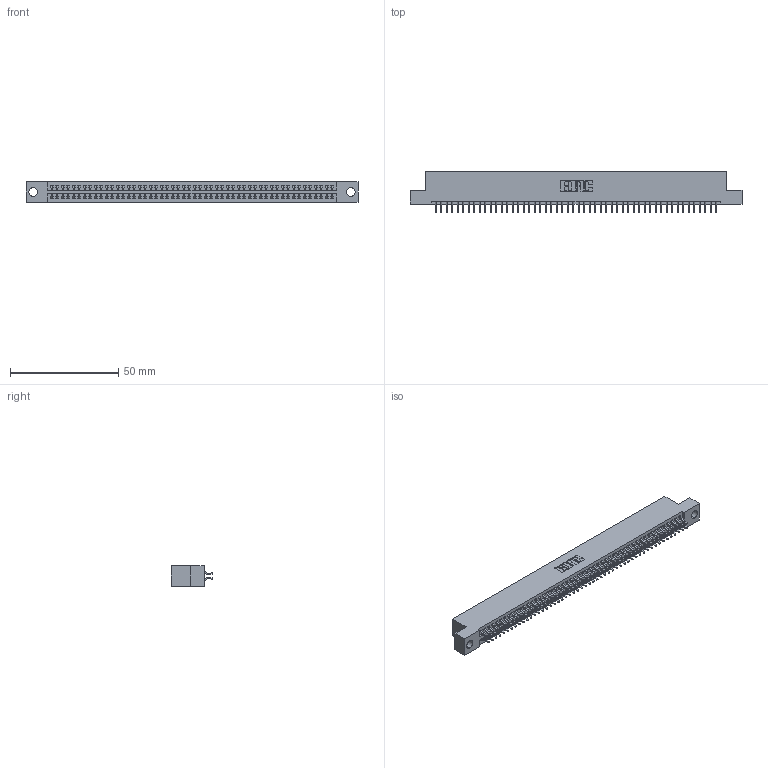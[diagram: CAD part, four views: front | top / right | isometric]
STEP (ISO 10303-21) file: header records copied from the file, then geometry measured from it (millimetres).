
FILE_DESCRIPTION (( 'STEP AP203' ), '1' );
FILE_NAME ('395-104-556-204.STEP', '2018-11-30T14:05:59', ( '' ), ( '' ), 'SwSTEP 2.0', 'SolidWorks 2016', '' );
FILE_SCHEMA (( 'CONFIG_CONTROL_DESIGN' ));
Length unit declared in the file: inch
Products named in the file (3): 395-104-556-204; 345 Part_Flush Mounting Lugs - 0.156 Dia-TH; 345-292-001_556 Tail
Assembly tree (105 placements, depth 2):
  395-104-556-204
    345 Part_Flush Mounting Lugs - 0.156 Dia-TH
    345-292-001_556 Tail  x104
Bounding box: 153.29 x 19.24 x 9.4 mm (x, y, z)
Volume: 14891.5 mm3; surface area: 21930 mm2
Topology: 105 solids, 105 shells, 5950 faces, 17709 edges, 11666 vertices
Faces by surface type: plane 3928, cylinder 2022
Entity records: 39677 total; most frequent: CARTESIAN_POINT 6656, ORIENTED_EDGE 6578, DIRECTION 5845, EDGE_CURVE 3289, VECTOR 2941, LINE 2941, VERTEX_POINT 2190, AXIS2_PLACEMENT_3D 1452
